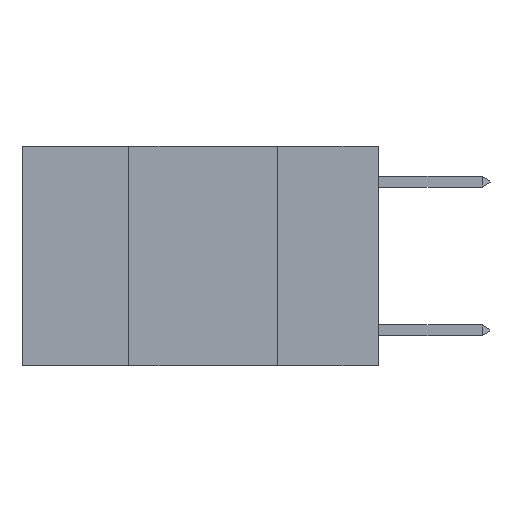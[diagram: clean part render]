
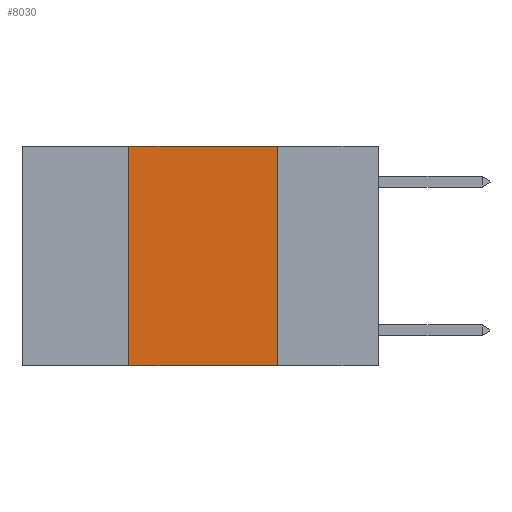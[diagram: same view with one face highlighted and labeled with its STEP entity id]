
A CAD part, left-side view. The second image highlights one B-rep face of the part: STEP entity #8030.
In plain terms, the highlighted planar face has unit normal (-1, 0, 0).
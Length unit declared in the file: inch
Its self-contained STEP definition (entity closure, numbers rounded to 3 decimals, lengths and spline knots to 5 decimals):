
#318 = CARTESIAN_POINT ( 'NONE',  ( 0., 0.6, -0.37 ) ) ;
#594 = CARTESIAN_POINT ( 'NONE',  ( 0., 0.17, 0. ) ) ;
#668 = DIRECTION ( 'NONE',  ( 0., -1., 0. ) ) ;
#1323 = LINE ( 'NONE', #4469, #22753 ) ;
#1702 = EDGE_CURVE ( 'NONE', #14343, #20614, #19804, .T. ) ;
#2264 = CARTESIAN_POINT ( 'NONE',  ( 0., 0.17, -0.37 ) ) ;
#2304 = DIRECTION ( 'NONE',  ( 0., -1., 0. ) ) ;
#3596 = VECTOR ( 'NONE', #668, 39.37008 ) ;
#3812 = VERTEX_POINT ( 'NONE', #24461 ) ;
#4469 = CARTESIAN_POINT ( 'NONE',  ( 0., 0.42, 0. ) ) ;
#5545 = EDGE_CURVE ( 'NONE', #6213, #20614, #20241, .T. ) ;
#6213 = VERTEX_POINT ( 'NONE', #18212 ) ;
#8030 = ADVANCED_FACE ( 'NONE', ( #8205 ), #16204, .F. ) ;
#8205 = FACE_OUTER_BOUND ( 'NONE', #21429, .T. ) ;
#8993 = ORIENTED_EDGE ( 'NONE', *, *, #19475, .F. ) ;
#12962 = CARTESIAN_POINT ( 'NONE',  ( 0., 0.6, 0. ) ) ;
#13306 = ORIENTED_EDGE ( 'NONE', *, *, #5545, .T. ) ;
#14343 = VERTEX_POINT ( 'NONE', #594 ) ;
#14421 = VECTOR ( 'NONE', #21704, 39.37008 ) ;
#15496 = EDGE_CURVE ( 'NONE', #3812, #14343, #20794, .T. ) ;
#15497 = DIRECTION ( 'NONE',  ( 0., 0., -1. ) ) ;
#15522 = DIRECTION ( 'NONE',  ( 1., 0., 0. ) ) ;
#15617 = CARTESIAN_POINT ( 'NONE',  ( 0., 0.6, 0. ) ) ;
#16204 = PLANE ( 'NONE',  #19667 ) ;
#17259 = ORIENTED_EDGE ( 'NONE', *, *, #15496, .F. ) ;
#18212 = CARTESIAN_POINT ( 'NONE',  ( 0., 0.42, -0.37 ) ) ;
#19475 = EDGE_CURVE ( 'NONE', #6213, #3812, #1323, .T. ) ;
#19667 = AXIS2_PLACEMENT_3D ( 'NONE', #15617, #15522, #15497 ) ;
#19804 = LINE ( 'NONE', #21885, #14421 ) ;
#20241 = LINE ( 'NONE', #318, #3596 ) ;
#20614 = VERTEX_POINT ( 'NONE', #2264 ) ;
#20794 = LINE ( 'NONE', #12962, #21407 ) ;
#21094 = DIRECTION ( 'NONE',  ( 0., 0., 1. ) ) ;
#21407 = VECTOR ( 'NONE', #2304, 39.37008 ) ;
#21429 = EDGE_LOOP ( 'NONE', ( #25924, #17259, #8993, #13306 ) ) ;
#21704 = DIRECTION ( 'NONE',  ( 0., 0., -1. ) ) ;
#21885 = CARTESIAN_POINT ( 'NONE',  ( 0., 0.17, 0. ) ) ;
#22753 = VECTOR ( 'NONE', #21094, 39.37008 ) ;
#24461 = CARTESIAN_POINT ( 'NONE',  ( 0., 0.42, 0. ) ) ;
#25924 = ORIENTED_EDGE ( 'NONE', *, *, #1702, .F. ) ;
